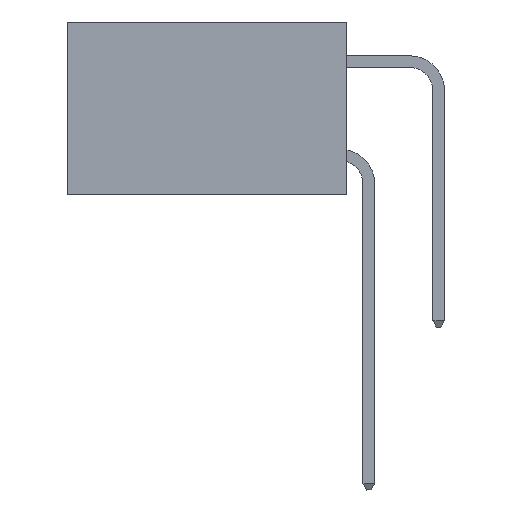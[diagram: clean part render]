
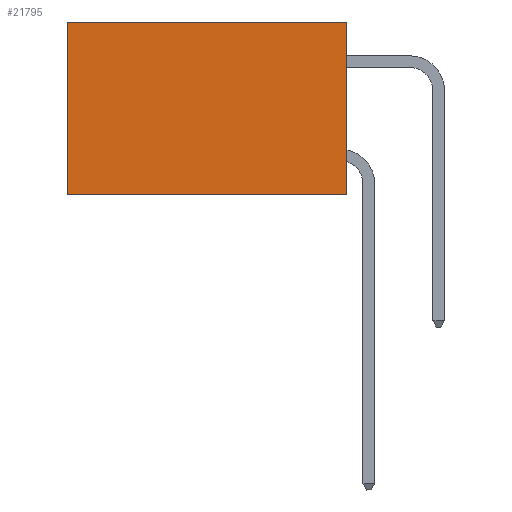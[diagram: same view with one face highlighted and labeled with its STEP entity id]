
A CAD part, left-side view. The second image highlights one B-rep face of the part: STEP entity #21795.
In plain terms, the highlighted planar face has unit normal (-1, 0, 0).
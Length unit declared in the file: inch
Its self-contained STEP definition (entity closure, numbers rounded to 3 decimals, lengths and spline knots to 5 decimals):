
#383 = CARTESIAN_POINT ( 'NONE',  ( 0.2875, 0.6, 0. ) ) ;
#988 = VERTEX_POINT ( 'NONE', #383 ) ;
#1875 = EDGE_LOOP ( 'NONE', ( #7089, #4656, #13405, #11863 ) ) ;
#1903 = CARTESIAN_POINT ( 'NONE',  ( 0.2875, 0.6, -0.37 ) ) ;
#1926 = LINE ( 'NONE', #6877, #20527 ) ;
#1993 = CARTESIAN_POINT ( 'NONE',  ( 0.2875, 0., -0.37 ) ) ;
#2074 = CARTESIAN_POINT ( 'NONE',  ( 0.2875, 0., 0. ) ) ;
#2655 = LINE ( 'NONE', #7915, #7582 ) ;
#2814 = VERTEX_POINT ( 'NONE', #1903 ) ;
#3142 = DIRECTION ( 'NONE',  ( 0., 0., -1. ) ) ;
#3775 = CARTESIAN_POINT ( 'NONE',  ( 0.2875, 0., 0. ) ) ;
#4656 = ORIENTED_EDGE ( 'NONE', *, *, #22137, .F. ) ;
#5373 = VERTEX_POINT ( 'NONE', #1993 ) ;
#5628 = PLANE ( 'NONE',  #21979 ) ;
#6560 = CARTESIAN_POINT ( 'NONE',  ( 0.2875, 0., -0.37 ) ) ;
#6877 = CARTESIAN_POINT ( 'NONE',  ( 0.2875, 0.6, 0. ) ) ;
#7089 = ORIENTED_EDGE ( 'NONE', *, *, #16291, .T. ) ;
#7582 = VECTOR ( 'NONE', #20368, 39.37008 ) ;
#7627 = VECTOR ( 'NONE', #13750, 39.37008 ) ;
#7915 = CARTESIAN_POINT ( 'NONE',  ( 0.2875, 0., 0. ) ) ;
#9250 = DIRECTION ( 'NONE',  ( 0., 0., -1. ) ) ;
#9500 = EDGE_CURVE ( 'NONE', #21749, #988, #2655, .T. ) ;
#9824 = FACE_OUTER_BOUND ( 'NONE', #1875, .T. ) ;
#11863 = ORIENTED_EDGE ( 'NONE', *, *, #9500, .T. ) ;
#12686 = CARTESIAN_POINT ( 'NONE',  ( 0.2875, 0., 0. ) ) ;
#13405 = ORIENTED_EDGE ( 'NONE', *, *, #16549, .F. ) ;
#13750 = DIRECTION ( 'NONE',  ( 0., 1., 0. ) ) ;
#14978 = VECTOR ( 'NONE', #16561, 39.37008 ) ;
#15520 = LINE ( 'NONE', #2074, #14978 ) ;
#16291 = EDGE_CURVE ( 'NONE', #988, #2814, #1926, .T. ) ;
#16549 = EDGE_CURVE ( 'NONE', #21749, #5373, #15520, .T. ) ;
#16561 = DIRECTION ( 'NONE',  ( 0., 0., -1. ) ) ;
#17102 = LINE ( 'NONE', #6560, #7627 ) ;
#19927 = DIRECTION ( 'NONE',  ( 1., 0., 0. ) ) ;
#20368 = DIRECTION ( 'NONE',  ( 0., 1., 0. ) ) ;
#20527 = VECTOR ( 'NONE', #3142, 39.37008 ) ;
#21749 = VERTEX_POINT ( 'NONE', #12686 ) ;
#21795 = ADVANCED_FACE ( 'NONE', ( #9824 ), #5628, .F. ) ;
#21979 = AXIS2_PLACEMENT_3D ( 'NONE', #3775, #19927, #9250 ) ;
#22137 = EDGE_CURVE ( 'NONE', #5373, #2814, #17102, .T. ) ;
